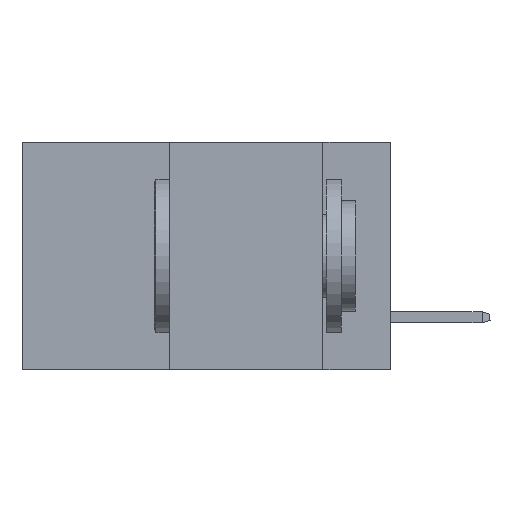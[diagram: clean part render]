
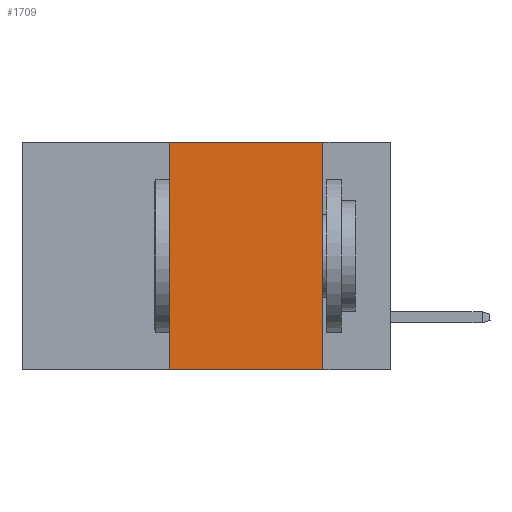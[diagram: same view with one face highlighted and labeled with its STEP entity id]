
A CAD part, left-side view. The second image highlights one B-rep face of the part: STEP entity #1709.
In plain terms, the highlighted planar face has unit normal (-1, 0, 0).
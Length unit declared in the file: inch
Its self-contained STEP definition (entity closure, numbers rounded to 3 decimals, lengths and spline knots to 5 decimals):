
#557 = EDGE_CURVE ( 'NONE', #7278, #863, #3242, .T. ) ;
#863 = VERTEX_POINT ( 'NONE', #2008 ) ;
#885 = CARTESIAN_POINT ( 'NONE',  ( 0., 0.6, -0.37 ) ) ;
#1638 = LINE ( 'NONE', #10782, #2113 ) ;
#1709 = ADVANCED_FACE ( 'NONE', ( #11542 ), #8960, .F. ) ;
#2008 = CARTESIAN_POINT ( 'NONE',  ( 0., 0.11, -0.37 ) ) ;
#2113 = VECTOR ( 'NONE', #3905, 39.37008 ) ;
#2505 = CARTESIAN_POINT ( 'NONE',  ( 0., 0.11, 0. ) ) ;
#2605 = ORIENTED_EDGE ( 'NONE', *, *, #11129, .F. ) ;
#3072 = DIRECTION ( 'NONE',  ( 1., 0., 0. ) ) ;
#3097 = VECTOR ( 'NONE', #10212, 39.37008 ) ;
#3156 = DIRECTION ( 'NONE',  ( 0., 0., -1. ) ) ;
#3242 = LINE ( 'NONE', #7253, #3097 ) ;
#3349 = DIRECTION ( 'NONE',  ( 0., 0., 1. ) ) ;
#3905 = DIRECTION ( 'NONE',  ( 0., -1., 0. ) ) ;
#4156 = VECTOR ( 'NONE', #5795, 39.37008 ) ;
#5795 = DIRECTION ( 'NONE',  ( 0., -1., 0. ) ) ;
#6418 = LINE ( 'NONE', #7130, #11209 ) ;
#6661 = VERTEX_POINT ( 'NONE', #10149 ) ;
#7130 = CARTESIAN_POINT ( 'NONE',  ( 0., 0.36, 0. ) ) ;
#7246 = EDGE_CURVE ( 'NONE', #6661, #7278, #1638, .T. ) ;
#7253 = CARTESIAN_POINT ( 'NONE',  ( 0., 0.11, 0. ) ) ;
#7278 = VERTEX_POINT ( 'NONE', #2505 ) ;
#7387 = CARTESIAN_POINT ( 'NONE',  ( 0., 0.36, -0.37 ) ) ;
#7583 = AXIS2_PLACEMENT_3D ( 'NONE', #12049, #3072, #3156 ) ;
#7642 = EDGE_LOOP ( 'NONE', ( #8874, #11161, #2605, #12674 ) ) ;
#8874 = ORIENTED_EDGE ( 'NONE', *, *, #557, .F. ) ;
#8960 = PLANE ( 'NONE',  #7583 ) ;
#9035 = EDGE_CURVE ( 'NONE', #9815, #863, #11108, .T. ) ;
#9815 = VERTEX_POINT ( 'NONE', #7387 ) ;
#10149 = CARTESIAN_POINT ( 'NONE',  ( 0., 0.36, 0. ) ) ;
#10212 = DIRECTION ( 'NONE',  ( 0., 0., -1. ) ) ;
#10782 = CARTESIAN_POINT ( 'NONE',  ( 0., 0.6, 0. ) ) ;
#11108 = LINE ( 'NONE', #885, #4156 ) ;
#11129 = EDGE_CURVE ( 'NONE', #9815, #6661, #6418, .T. ) ;
#11161 = ORIENTED_EDGE ( 'NONE', *, *, #7246, .F. ) ;
#11209 = VECTOR ( 'NONE', #3349, 39.37008 ) ;
#11542 = FACE_OUTER_BOUND ( 'NONE', #7642, .T. ) ;
#12049 = CARTESIAN_POINT ( 'NONE',  ( 0., 0.6, 0. ) ) ;
#12674 = ORIENTED_EDGE ( 'NONE', *, *, #9035, .T. ) ;
